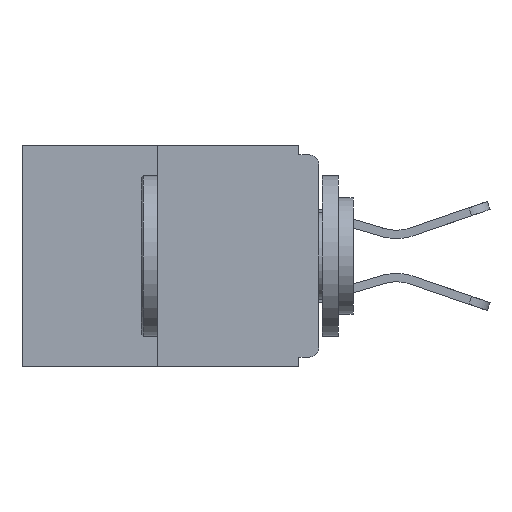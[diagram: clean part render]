
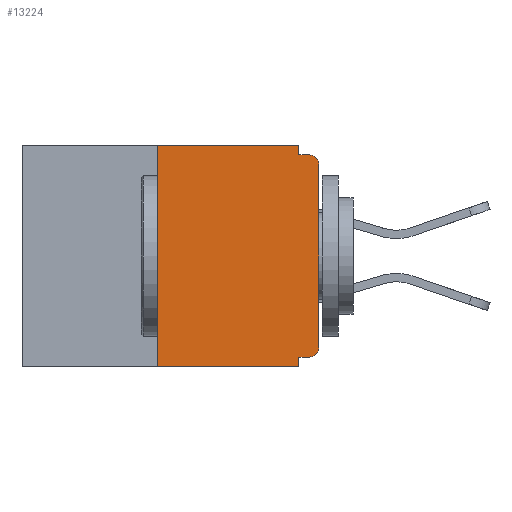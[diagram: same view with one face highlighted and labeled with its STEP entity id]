
A CAD part, left-side view. The second image highlights one B-rep face of the part: STEP entity #13224.
In plain terms, the highlighted planar face has unit normal (-1, 0, 0).
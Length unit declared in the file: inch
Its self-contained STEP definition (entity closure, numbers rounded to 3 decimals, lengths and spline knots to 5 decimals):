
#33 = CARTESIAN_POINT ( 'NONE',  ( 0., 0.25, 0. ) ) ;
#672 = EDGE_LOOP ( 'NONE', ( #16680, #21716, #25057, #27517, #6999, #14642, #23828, #10983, #27298, #2460 ) ) ;
#845 = CARTESIAN_POINT ( 'NONE',  ( 0., 0.031, -0.328 ) ) ;
#1540 = LINE ( 'NONE', #18686, #12354 ) ;
#2051 = VECTOR ( 'NONE', #12030, 39.37008 ) ;
#2054 = VERTEX_POINT ( 'NONE', #15966 ) ;
#2460 = ORIENTED_EDGE ( 'NONE', *, *, #16356, .F. ) ;
#2560 = CARTESIAN_POINT ( 'NONE',  ( 0., 0.015, -0.03 ) ) ;
#2934 = VERTEX_POINT ( 'NONE', #11054 ) ;
#2953 = LINE ( 'NONE', #15843, #10778 ) ;
#4692 = VERTEX_POINT ( 'NONE', #9986 ) ;
#4707 = DIRECTION ( 'NONE',  ( 0., 0., -1. ) ) ;
#4821 = DIRECTION ( 'NONE',  ( 0., 0., -1. ) ) ;
#5409 = LINE ( 'NONE', #27037, #14914 ) ;
#5412 = CARTESIAN_POINT ( 'NONE',  ( 0., 0.031, -0.015 ) ) ;
#5738 = CARTESIAN_POINT ( 'NONE',  ( 0., 0.25, -0.343 ) ) ;
#5810 = VECTOR ( 'NONE', #18125, 39.37008 ) ;
#5878 = CIRCLE ( 'NONE', #13701, 0.015 ) ;
#5978 = VERTEX_POINT ( 'NONE', #845 ) ;
#6067 = EDGE_CURVE ( 'NONE', #19045, #2054, #9240, .T. ) ;
#6087 = DIRECTION ( 'NONE',  ( -1., 0., 0. ) ) ;
#6233 = CARTESIAN_POINT ( 'NONE',  ( 0., 0.015, -0.328 ) ) ;
#6741 = EDGE_CURVE ( 'NONE', #19045, #9254, #25800, .T. ) ;
#6929 = EDGE_CURVE ( 'NONE', #23771, #5978, #16634, .T. ) ;
#6999 = ORIENTED_EDGE ( 'NONE', *, *, #6929, .F. ) ;
#7104 = DIRECTION ( 'NONE',  ( 0., 1., 0. ) ) ;
#7150 = DIRECTION ( 'NONE',  ( 0., -1., 0. ) ) ;
#7274 = CIRCLE ( 'NONE', #22209, 0.015 ) ;
#7506 = VERTEX_POINT ( 'NONE', #16160 ) ;
#7939 = DIRECTION ( 'NONE',  ( 0., 0., -1. ) ) ;
#8278 = DIRECTION ( 'NONE',  ( 0., 0., -1. ) ) ;
#8717 = DIRECTION ( 'NONE',  ( 1., 0., 0. ) ) ;
#8933 = DIRECTION ( 'NONE',  ( 0., 0., -1. ) ) ;
#9240 = LINE ( 'NONE', #24918, #11292 ) ;
#9254 = VERTEX_POINT ( 'NONE', #33 ) ;
#9443 = CARTESIAN_POINT ( 'NONE',  ( 0., 0., -0.313 ) ) ;
#9832 = CARTESIAN_POINT ( 'NONE',  ( 0., 0.25, 0. ) ) ;
#9986 = CARTESIAN_POINT ( 'NONE',  ( 0., 0.015, -0.015 ) ) ;
#10778 = VECTOR ( 'NONE', #7150, 39.37008 ) ;
#10983 = ORIENTED_EDGE ( 'NONE', *, *, #17506, .T. ) ;
#11054 = CARTESIAN_POINT ( 'NONE',  ( 0., 0.031, 0. ) ) ;
#11292 = VECTOR ( 'NONE', #20660, 39.37008 ) ;
#11507 = EDGE_CURVE ( 'NONE', #12310, #4692, #26154, .T. ) ;
#12030 = DIRECTION ( 'NONE',  ( 0., 0., 1. ) ) ;
#12310 = VERTEX_POINT ( 'NONE', #5412 ) ;
#12354 = VECTOR ( 'NONE', #7939, 39.37008 ) ;
#12808 = EDGE_CURVE ( 'NONE', #13265, #7506, #26725, .T. ) ;
#13092 = AXIS2_PLACEMENT_3D ( 'NONE', #22024, #8717, #4707 ) ;
#13224 = ADVANCED_FACE ( 'NONE', ( #20613 ), #26280, .F. ) ;
#13265 = VERTEX_POINT ( 'NONE', #9443 ) ;
#13701 = AXIS2_PLACEMENT_3D ( 'NONE', #2560, #21870, #8933 ) ;
#14642 = ORIENTED_EDGE ( 'NONE', *, *, #15945, .T. ) ;
#14914 = VECTOR ( 'NONE', #4821, 39.37008 ) ;
#15843 = CARTESIAN_POINT ( 'NONE',  ( 0., 0.46, 0. ) ) ;
#15945 = EDGE_CURVE ( 'NONE', #23771, #13265, #7274, .T. ) ;
#15966 = CARTESIAN_POINT ( 'NONE',  ( 0., 0.031, -0.343 ) ) ;
#16160 = CARTESIAN_POINT ( 'NONE',  ( 0., 0., -0.03 ) ) ;
#16356 = EDGE_CURVE ( 'NONE', #2934, #12310, #1540, .T. ) ;
#16634 = LINE ( 'NONE', #22070, #20341 ) ;
#16680 = ORIENTED_EDGE ( 'NONE', *, *, #20706, .F. ) ;
#17506 = EDGE_CURVE ( 'NONE', #7506, #4692, #5878, .T. ) ;
#18125 = DIRECTION ( 'NONE',  ( 0., 0., 1. ) ) ;
#18686 = CARTESIAN_POINT ( 'NONE',  ( 0., 0.031, 0. ) ) ;
#19013 = CARTESIAN_POINT ( 'NONE',  ( 0., 0.015, -0.313 ) ) ;
#19045 = VERTEX_POINT ( 'NONE', #5738 ) ;
#19329 = EDGE_CURVE ( 'NONE', #5978, #2054, #5409, .T. ) ;
#20341 = VECTOR ( 'NONE', #7104, 39.37008 ) ;
#20613 = FACE_OUTER_BOUND ( 'NONE', #672, .T. ) ;
#20660 = DIRECTION ( 'NONE',  ( 0., -1., 0. ) ) ;
#20706 = EDGE_CURVE ( 'NONE', #9254, #2934, #2953, .T. ) ;
#21716 = ORIENTED_EDGE ( 'NONE', *, *, #6741, .F. ) ;
#21768 = VECTOR ( 'NONE', #22126, 39.37008 ) ;
#21870 = DIRECTION ( 'NONE',  ( -1., 0., 0. ) ) ;
#22024 = CARTESIAN_POINT ( 'NONE',  ( 0., 0.46, 0. ) ) ;
#22030 = CARTESIAN_POINT ( 'NONE',  ( 0., 0., -0.015 ) ) ;
#22070 = CARTESIAN_POINT ( 'NONE',  ( 0., 0., -0.328 ) ) ;
#22126 = DIRECTION ( 'NONE',  ( 0., -1., 0. ) ) ;
#22209 = AXIS2_PLACEMENT_3D ( 'NONE', #19013, #6087, #8278 ) ;
#22712 = CARTESIAN_POINT ( 'NONE',  ( 0., 0., 0. ) ) ;
#23771 = VERTEX_POINT ( 'NONE', #6233 ) ;
#23828 = ORIENTED_EDGE ( 'NONE', *, *, #12808, .T. ) ;
#24918 = CARTESIAN_POINT ( 'NONE',  ( 0., 0.46, -0.343 ) ) ;
#25057 = ORIENTED_EDGE ( 'NONE', *, *, #6067, .T. ) ;
#25800 = LINE ( 'NONE', #9832, #5810 ) ;
#26154 = LINE ( 'NONE', #22030, #21768 ) ;
#26280 = PLANE ( 'NONE',  #13092 ) ;
#26725 = LINE ( 'NONE', #22712, #2051 ) ;
#27037 = CARTESIAN_POINT ( 'NONE',  ( 0., 0.031, -0.343 ) ) ;
#27298 = ORIENTED_EDGE ( 'NONE', *, *, #11507, .F. ) ;
#27517 = ORIENTED_EDGE ( 'NONE', *, *, #19329, .F. ) ;
